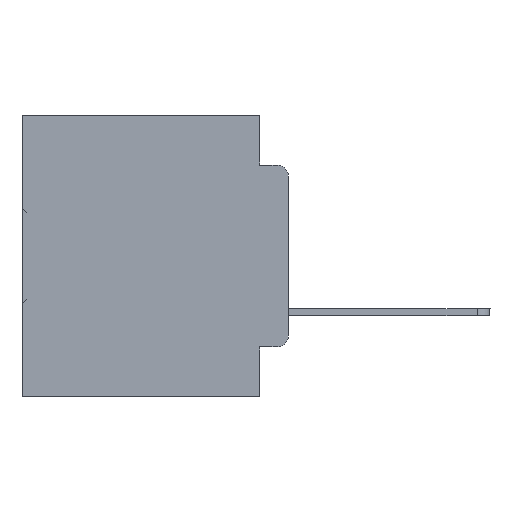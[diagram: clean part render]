
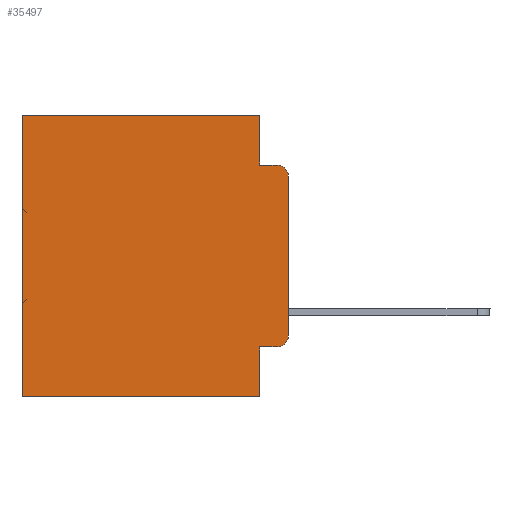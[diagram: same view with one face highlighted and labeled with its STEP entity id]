
A CAD part, left-side view. The second image highlights one B-rep face of the part: STEP entity #35497.
In plain terms, the highlighted planar face has unit normal (-1, 0, 0).
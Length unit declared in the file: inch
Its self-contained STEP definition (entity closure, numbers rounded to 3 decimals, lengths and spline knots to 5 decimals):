
#57 = DIRECTION ( 'NONE',  ( 0., 0., -1. ) ) ;
#177 = EDGE_CURVE ( 'NONE', #11537, #27466, #31905, .T. ) ;
#1248 = ORIENTED_EDGE ( 'NONE', *, *, #18314, .F. ) ;
#1736 = LINE ( 'NONE', #4986, #31746 ) ;
#1806 = CARTESIAN_POINT ( 'NONE',  ( 0.298, 0.051, -0.0885 ) ) ;
#2208 = VECTOR ( 'NONE', #35395, 39.37008 ) ;
#3426 = VERTEX_POINT ( 'NONE', #10644 ) ;
#3429 = CARTESIAN_POINT ( 'NONE',  ( 0.298, 0.051, 0. ) ) ;
#3808 = CARTESIAN_POINT ( 'NONE',  ( 0.298, 0., 0. ) ) ;
#4536 = VERTEX_POINT ( 'NONE', #1806 ) ;
#4986 = CARTESIAN_POINT ( 'NONE',  ( 0.298, 0.473, 0. ) ) ;
#5205 = EDGE_CURVE ( 'NONE', #5572, #3426, #16886, .T. ) ;
#5376 = DIRECTION ( 'NONE',  ( -1., 0., 0. ) ) ;
#5572 = VERTEX_POINT ( 'NONE', #14776 ) ;
#5856 = EDGE_CURVE ( 'NONE', #22267, #4536, #36553, .T. ) ;
#5937 = CARTESIAN_POINT ( 'NONE',  ( 0.298, 0.02, -0.0885 ) ) ;
#6180 = CARTESIAN_POINT ( 'NONE',  ( 0.298, 0., -0.3915 ) ) ;
#6668 = ORIENTED_EDGE ( 'NONE', *, *, #12971, .F. ) ;
#7196 = LINE ( 'NONE', #35411, #21546 ) ;
#7197 = DIRECTION ( 'NONE',  ( 0., -1., 0. ) ) ;
#7430 = VECTOR ( 'NONE', #32970, 39.37008 ) ;
#7538 = VECTOR ( 'NONE', #33690, 39.37008 ) ;
#7723 = CARTESIAN_POINT ( 'NONE',  ( 0.298, 0.473, -0.5 ) ) ;
#7885 = LINE ( 'NONE', #3429, #10607 ) ;
#7945 = DIRECTION ( 'NONE',  ( 1., 0., 0. ) ) ;
#8212 = ORIENTED_EDGE ( 'NONE', *, *, #23640, .F. ) ;
#8264 = AXIS2_PLACEMENT_3D ( 'NONE', #22880, #23267, #57 ) ;
#8748 = ORIENTED_EDGE ( 'NONE', *, *, #19270, .F. ) ;
#8851 = LINE ( 'NONE', #36543, #28633 ) ;
#9291 = DIRECTION ( 'NONE',  ( 0., 0., -1. ) ) ;
#10607 = VECTOR ( 'NONE', #9291, 39.37008 ) ;
#10644 = CARTESIAN_POINT ( 'NONE',  ( 0.298, 0.02, -0.4115 ) ) ;
#10680 = EDGE_CURVE ( 'NONE', #3426, #32155, #16776, .T. ) ;
#11537 = VERTEX_POINT ( 'NONE', #12969 ) ;
#11857 = VECTOR ( 'NONE', #24402, 39.37008 ) ;
#12087 = CARTESIAN_POINT ( 'NONE',  ( 0.298, 0.473, 0. ) ) ;
#12969 = CARTESIAN_POINT ( 'NONE',  ( 0.298, 0., -0.1085 ) ) ;
#12971 = EDGE_CURVE ( 'NONE', #4536, #27466, #7196, .T. ) ;
#13602 = DIRECTION ( 'NONE',  ( 0., 0., -1. ) ) ;
#13803 = ORIENTED_EDGE ( 'NONE', *, *, #177, .T. ) ;
#13961 = DIRECTION ( 'NONE',  ( 0., 1., 0. ) ) ;
#14776 = CARTESIAN_POINT ( 'NONE',  ( 0.298, 0.051, -0.4115 ) ) ;
#14890 = AXIS2_PLACEMENT_3D ( 'NONE', #22563, #5376, #18459 ) ;
#15739 = VERTEX_POINT ( 'NONE', #7723 ) ;
#16776 = CIRCLE ( 'NONE', #14890, 0.02 ) ;
#16886 = LINE ( 'NONE', #21710, #7430 ) ;
#17823 = ORIENTED_EDGE ( 'NONE', *, *, #5205, .T. ) ;
#18314 = EDGE_CURVE ( 'NONE', #36515, #15739, #27751, .T. ) ;
#18459 = DIRECTION ( 'NONE',  ( 0., 0., -1. ) ) ;
#18986 = EDGE_CURVE ( 'NONE', #22267, #35971, #8851, .T. ) ;
#19195 = DIRECTION ( 'NONE',  ( 0., 0., -1. ) ) ;
#19270 = EDGE_CURVE ( 'NONE', #5572, #36515, #7885, .T. ) ;
#19445 = CARTESIAN_POINT ( 'NONE',  ( 0.298, 0., -0.5 ) ) ;
#21546 = VECTOR ( 'NONE', #7197, 39.37008 ) ;
#21710 = CARTESIAN_POINT ( 'NONE',  ( 0.298, 0.051, -0.4115 ) ) ;
#22267 = VERTEX_POINT ( 'NONE', #26208 ) ;
#22563 = CARTESIAN_POINT ( 'NONE',  ( 0.298, 0.02, -0.3915 ) ) ;
#22880 = CARTESIAN_POINT ( 'NONE',  ( 0.298, 0.02, -0.1085 ) ) ;
#23267 = DIRECTION ( 'NONE',  ( -1., 0., 0. ) ) ;
#23540 = FACE_OUTER_BOUND ( 'NONE', #27186, .T. ) ;
#23640 = EDGE_CURVE ( 'NONE', #11537, #32155, #32696, .T. ) ;
#24402 = DIRECTION ( 'NONE',  ( 0., 0., -1. ) ) ;
#25136 = CARTESIAN_POINT ( 'NONE',  ( 0.298, 0., 0. ) ) ;
#26208 = CARTESIAN_POINT ( 'NONE',  ( 0.298, 0.051, 0. ) ) ;
#26224 = AXIS2_PLACEMENT_3D ( 'NONE', #25136, #7945, #13602 ) ;
#27186 = EDGE_LOOP ( 'NONE', ( #8212, #13803, #6668, #36958, #33842, #32607, #1248, #8748, #17823, #36170 ) ) ;
#27466 = VERTEX_POINT ( 'NONE', #5937 ) ;
#27751 = LINE ( 'NONE', #19445, #7538 ) ;
#28633 = VECTOR ( 'NONE', #13961, 39.37008 ) ;
#31746 = VECTOR ( 'NONE', #19195, 39.37008 ) ;
#31905 = CIRCLE ( 'NONE', #8264, 0.02 ) ;
#32155 = VERTEX_POINT ( 'NONE', #6180 ) ;
#32607 = ORIENTED_EDGE ( 'NONE', *, *, #32777, .T. ) ;
#32618 = CARTESIAN_POINT ( 'NONE',  ( 0.298, 0.051, -0.5 ) ) ;
#32696 = LINE ( 'NONE', #3808, #2208 ) ;
#32777 = EDGE_CURVE ( 'NONE', #35971, #15739, #1736, .T. ) ;
#32970 = DIRECTION ( 'NONE',  ( 0., -1., 0. ) ) ;
#33690 = DIRECTION ( 'NONE',  ( 0., 1., 0. ) ) ;
#33842 = ORIENTED_EDGE ( 'NONE', *, *, #18986, .T. ) ;
#35395 = DIRECTION ( 'NONE',  ( 0., 0., -1. ) ) ;
#35411 = CARTESIAN_POINT ( 'NONE',  ( 0.298, 0.051, -0.0885 ) ) ;
#35497 = ADVANCED_FACE ( 'NONE', ( #23540 ), #36083, .F. ) ;
#35971 = VERTEX_POINT ( 'NONE', #12087 ) ;
#36083 = PLANE ( 'NONE',  #26224 ) ;
#36170 = ORIENTED_EDGE ( 'NONE', *, *, #10680, .T. ) ;
#36515 = VERTEX_POINT ( 'NONE', #32618 ) ;
#36543 = CARTESIAN_POINT ( 'NONE',  ( 0.298, 0., 0. ) ) ;
#36553 = LINE ( 'NONE', #36682, #11857 ) ;
#36682 = CARTESIAN_POINT ( 'NONE',  ( 0.298, 0.051, 0. ) ) ;
#36958 = ORIENTED_EDGE ( 'NONE', *, *, #5856, .F. ) ;
